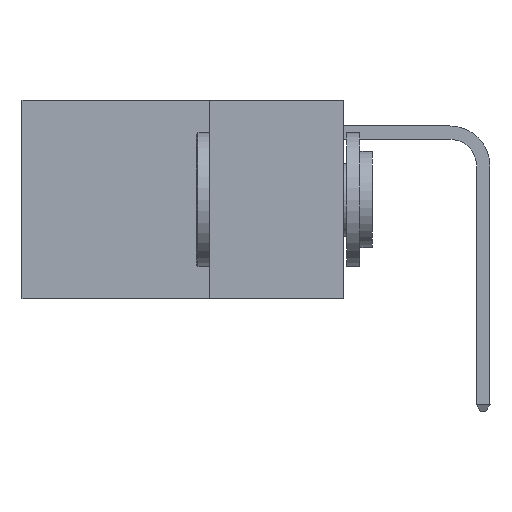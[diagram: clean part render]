
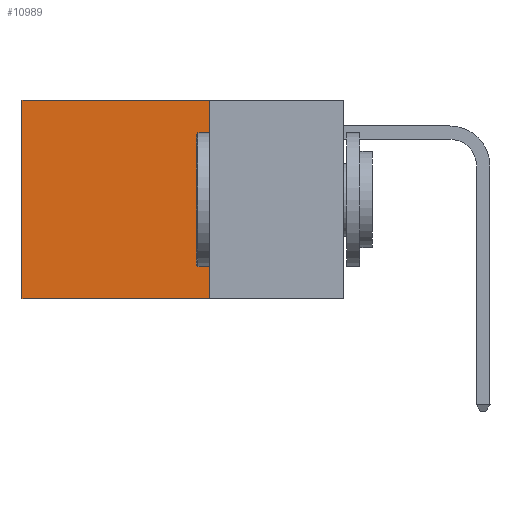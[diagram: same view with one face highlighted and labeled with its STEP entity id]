
A CAD part, left-side view. The second image highlights one B-rep face of the part: STEP entity #10989.
In plain terms, the highlighted planar face has unit normal (-1, 0, 0).
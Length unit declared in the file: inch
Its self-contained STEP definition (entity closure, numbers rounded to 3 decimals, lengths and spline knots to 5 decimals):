
#190 = VECTOR ( 'NONE', #16330, 39.37008 ) ;
#336 = DIRECTION ( 'NONE',  ( 0., 1., 0. ) ) ;
#453 = CARTESIAN_POINT ( 'NONE',  ( 0.2625, 0.6, 0. ) ) ;
#1156 = VERTEX_POINT ( 'NONE', #1679 ) ;
#1679 = CARTESIAN_POINT ( 'NONE',  ( 0.2625, 0.6, -0.37 ) ) ;
#2538 = CARTESIAN_POINT ( 'NONE',  ( 0.2625, 0.25, 0. ) ) ;
#4090 = EDGE_CURVE ( 'NONE', #27760, #11182, #18108, .T. ) ;
#4136 = EDGE_CURVE ( 'NONE', #11182, #1156, #14676, .T. ) ;
#5745 = DIRECTION ( 'NONE',  ( 0., 0., -1. ) ) ;
#9039 = VECTOR ( 'NONE', #5745, 39.37008 ) ;
#9186 = FACE_OUTER_BOUND ( 'NONE', #10528, .T. ) ;
#9279 = VERTEX_POINT ( 'NONE', #14590 ) ;
#10528 = EDGE_LOOP ( 'NONE', ( #16733, #16027, #15260, #26186 ) ) ;
#10989 = ADVANCED_FACE ( 'NONE', ( #9186 ), #15548, .F. ) ;
#11182 = VERTEX_POINT ( 'NONE', #453 ) ;
#11457 = DIRECTION ( 'NONE',  ( 0., 1., 0. ) ) ;
#12539 = CARTESIAN_POINT ( 'NONE',  ( 0.2625, 0.25, 0. ) ) ;
#13670 = CARTESIAN_POINT ( 'NONE',  ( 0.2625, 0.25, 0. ) ) ;
#13844 = VECTOR ( 'NONE', #11457, 39.37008 ) ;
#14590 = CARTESIAN_POINT ( 'NONE',  ( 0.2625, 0.25, -0.37 ) ) ;
#14676 = LINE ( 'NONE', #18681, #190 ) ;
#15260 = ORIENTED_EDGE ( 'NONE', *, *, #24766, .F. ) ;
#15407 = DIRECTION ( 'NONE',  ( 0., 0., -1. ) ) ;
#15548 = PLANE ( 'NONE',  #27571 ) ;
#16027 = ORIENTED_EDGE ( 'NONE', *, *, #24132, .F. ) ;
#16330 = DIRECTION ( 'NONE',  ( 0., 0., -1. ) ) ;
#16733 = ORIENTED_EDGE ( 'NONE', *, *, #4136, .T. ) ;
#18108 = LINE ( 'NONE', #13670, #13844 ) ;
#18681 = CARTESIAN_POINT ( 'NONE',  ( 0.2625, 0.6, 0. ) ) ;
#19183 = LINE ( 'NONE', #12539, #9039 ) ;
#20258 = DIRECTION ( 'NONE',  ( 1., 0., 0. ) ) ;
#20563 = CARTESIAN_POINT ( 'NONE',  ( 0.2625, 0.25, -0.37 ) ) ;
#22778 = LINE ( 'NONE', #20563, #24314 ) ;
#23458 = CARTESIAN_POINT ( 'NONE',  ( 0.2625, 0.25, 0. ) ) ;
#24132 = EDGE_CURVE ( 'NONE', #9279, #1156, #22778, .T. ) ;
#24314 = VECTOR ( 'NONE', #336, 39.37008 ) ;
#24766 = EDGE_CURVE ( 'NONE', #27760, #9279, #19183, .T. ) ;
#26186 = ORIENTED_EDGE ( 'NONE', *, *, #4090, .T. ) ;
#27571 = AXIS2_PLACEMENT_3D ( 'NONE', #2538, #20258, #15407 ) ;
#27760 = VERTEX_POINT ( 'NONE', #23458 ) ;
